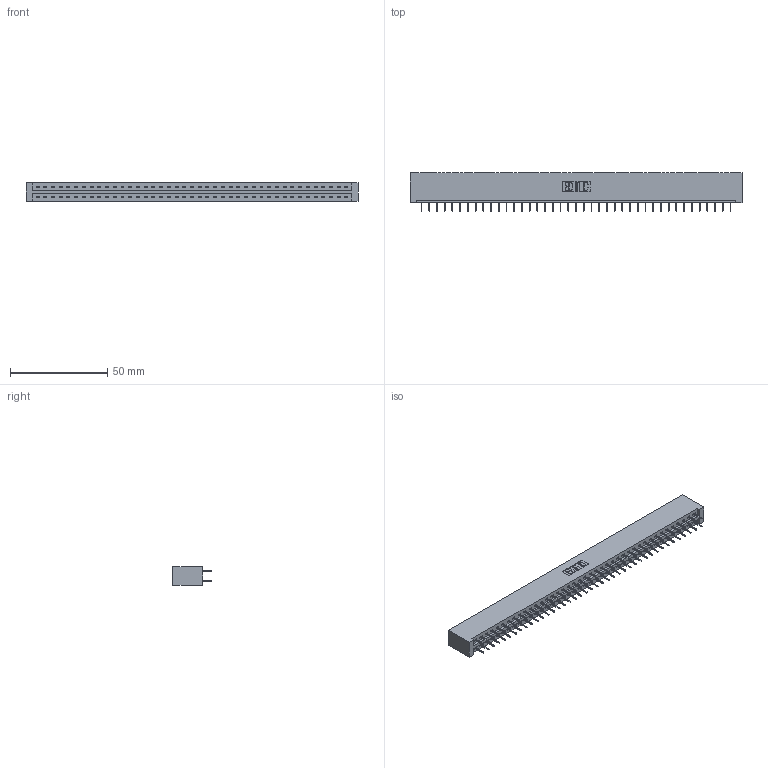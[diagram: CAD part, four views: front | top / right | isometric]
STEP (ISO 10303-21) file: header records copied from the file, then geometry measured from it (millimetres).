
FILE_DESCRIPTION (( 'STEP AP203' ), '1' );
FILE_NAME ('387-082-524-201.STEP', '2019-10-22T23:26:45', ( '' ), ( '' ), 'SwSTEP 2.0', 'SolidWorks 2016', '' );
FILE_SCHEMA (( 'CONFIG_CONTROL_DESIGN' ));
Length unit declared in the file: inch
Products named in the file (3): 345-292-001_345-293-124; 337 Part_No Mounting Lugs; 387-082-524-201
Assembly tree (83 placements, depth 2):
  387-082-524-201
    337 Part_No Mounting Lugs
    345-292-001_345-293-124  x82
Bounding box: 170.33 x 19.69 x 9.4 mm (x, y, z)
Volume: 18574.3 mm3; surface area: 20660.3 mm2
Topology: 83 solids, 83 shells, 4862 faces, 13817 edges, 8882 vertices
Faces by surface type: plane 3674, cylinder 1188
Entity records: 31715 total; most frequent: CARTESIAN_POINT 5342, ORIENTED_EDGE 5278, DIRECTION 4539, EDGE_CURVE 2639, VECTOR 2523, LINE 2523, VERTEX_POINT 1754, AXIS2_PLACEMENT_3D 1008
